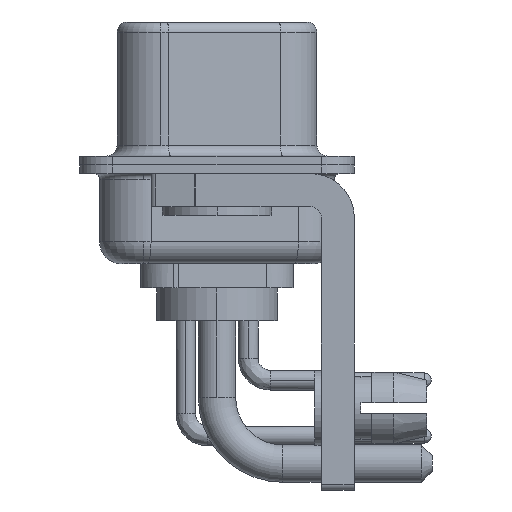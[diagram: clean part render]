
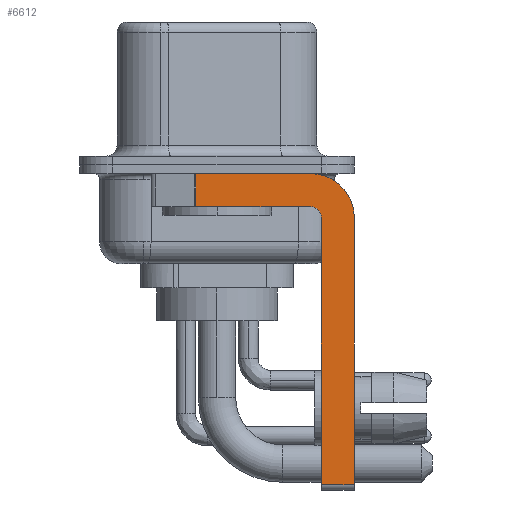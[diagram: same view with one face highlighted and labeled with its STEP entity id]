
A CAD part, left-side view. The second image highlights one B-rep face of the part: STEP entity #6612.
In plain terms, the highlighted planar face has unit normal (-1, 0, 0).
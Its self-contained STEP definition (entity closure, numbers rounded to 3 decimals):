
#338 = ORIENTED_EDGE ( 'NONE', *, *, #28988, .T. ) ;
#868 = VECTOR ( 'NONE', #25807, 1000. ) ;
#1048 = DIRECTION ( 'NONE',  ( 0., -1., 0. ) ) ;
#1994 = DIRECTION ( 'NONE',  ( 0., 0., -1. ) ) ;
#2663 = VERTEX_POINT ( 'NONE', #24443 ) ;
#2701 = CIRCLE ( 'NONE', #30660, 0.5 ) ;
#2788 = LINE ( 'NONE', #29220, #6670 ) ;
#3777 = CARTESIAN_POINT ( 'NONE',  ( -2.9, -4.25, -2.4 ) ) ;
#4065 = CARTESIAN_POINT ( 'NONE',  ( -2.9, -4.25, -1.9 ) ) ;
#4340 = ORIENTED_EDGE ( 'NONE', *, *, #30450, .F. ) ;
#4348 = VECTOR ( 'NONE', #19993, 1000. ) ;
#4601 = CARTESIAN_POINT ( 'NONE',  ( -2.9, -4.25, -0.4 ) ) ;
#5052 = CARTESIAN_POINT ( 'NONE',  ( -2.9, -4.25, -2.4 ) ) ;
#5652 = CIRCLE ( 'NONE', #23116, 2. ) ;
#6239 = DIRECTION ( 'NONE',  ( 1., 0., 0. ) ) ;
#6262 = VERTEX_POINT ( 'NONE', #14786 ) ;
#6302 = VERTEX_POINT ( 'NONE', #29773 ) ;
#6612 = ADVANCED_FACE ( 'NONE', ( #21775 ), #26008, .F. ) ;
#6670 = VECTOR ( 'NONE', #12960, 1000. ) ;
#8098 = LINE ( 'NONE', #15150, #29184 ) ;
#8377 = CARTESIAN_POINT ( 'NONE',  ( -2.9, -6.25, -2.4 ) ) ;
#8715 = ORIENTED_EDGE ( 'NONE', *, *, #28259, .F. ) ;
#8786 = DIRECTION ( 'NONE',  ( -1., 0., 0. ) ) ;
#9657 = VERTEX_POINT ( 'NONE', #15737 ) ;
#11607 = VECTOR ( 'NONE', #11825, 1000. ) ;
#11825 = DIRECTION ( 'NONE',  ( 0., 0., -1. ) ) ;
#11915 = DIRECTION ( 'NONE',  ( 0., 0., 1. ) ) ;
#12555 = CARTESIAN_POINT ( 'NONE',  ( -2.9, 0.978, -1.9 ) ) ;
#12960 = DIRECTION ( 'NONE',  ( 0., 0., -1. ) ) ;
#13123 = CARTESIAN_POINT ( 'NONE',  ( -2.9, -4.75, -14.8 ) ) ;
#13683 = ORIENTED_EDGE ( 'NONE', *, *, #20551, .T. ) ;
#14695 = DIRECTION ( 'NONE',  ( 0., -1., 0. ) ) ;
#14786 = CARTESIAN_POINT ( 'NONE',  ( -2.9, 0.978, -1.9 ) ) ;
#15150 = CARTESIAN_POINT ( 'NONE',  ( -2.9, 3., -0.4 ) ) ;
#15737 = CARTESIAN_POINT ( 'NONE',  ( -2.9, -4.25, -1.9 ) ) ;
#15927 = VERTEX_POINT ( 'NONE', #8377 ) ;
#16011 = EDGE_CURVE ( 'NONE', #9657, #6262, #25489, .T. ) ;
#16141 = CARTESIAN_POINT ( 'NONE',  ( -2.9, -6.25, -14.55 ) ) ;
#16448 = EDGE_CURVE ( 'NONE', #6302, #2663, #24690, .T. ) ;
#17642 = CARTESIAN_POINT ( 'NONE',  ( -2.9, -4.25, -14.55 ) ) ;
#18963 = DIRECTION ( 'NONE',  ( 1., 0., 0. ) ) ;
#19993 = DIRECTION ( 'NONE',  ( 0., 0., 1. ) ) ;
#20482 = VECTOR ( 'NONE', #1048, 1000. ) ;
#20551 = EDGE_CURVE ( 'NONE', #6302, #25291, #25135, .T. ) ;
#21337 = VERTEX_POINT ( 'NONE', #4601 ) ;
#21468 = DIRECTION ( 'NONE',  ( 0., 0., -1. ) ) ;
#21503 = ORIENTED_EDGE ( 'NONE', *, *, #25377, .F. ) ;
#21775 = FACE_OUTER_BOUND ( 'NONE', #22933, .T. ) ;
#22260 = CARTESIAN_POINT ( 'NONE',  ( -2.9, 0.978, -0.4 ) ) ;
#22804 = CARTESIAN_POINT ( 'NONE',  ( -2.9, -4.25, -2.4 ) ) ;
#22933 = EDGE_LOOP ( 'NONE', ( #29993, #338, #24516, #21503, #29927, #13683, #4340, #8715 ) ) ;
#23116 = AXIS2_PLACEMENT_3D ( 'NONE', #22804, #6239, #1994 ) ;
#24443 = CARTESIAN_POINT ( 'NONE',  ( -2.9, -4.75, -2.4 ) ) ;
#24516 = ORIENTED_EDGE ( 'NONE', *, *, #16011, .F. ) ;
#24690 = LINE ( 'NONE', #13123, #4348 ) ;
#25135 = LINE ( 'NONE', #17642, #20482 ) ;
#25291 = VERTEX_POINT ( 'NONE', #16141 ) ;
#25377 = EDGE_CURVE ( 'NONE', #2663, #9657, #2701, .T. ) ;
#25408 = AXIS2_PLACEMENT_3D ( 'NONE', #5052, #18963, #21468 ) ;
#25489 = LINE ( 'NONE', #4065, #868 ) ;
#25807 = DIRECTION ( 'NONE',  ( 0., 1., 0. ) ) ;
#26008 = PLANE ( 'NONE',  #25408 ) ;
#27222 = VERTEX_POINT ( 'NONE', #22260 ) ;
#28259 = EDGE_CURVE ( 'NONE', #21337, #15927, #5652, .T. ) ;
#28988 = EDGE_CURVE ( 'NONE', #27222, #6262, #30595, .T. ) ;
#29184 = VECTOR ( 'NONE', #14695, 1000. ) ;
#29220 = CARTESIAN_POINT ( 'NONE',  ( -2.9, -6.25, -2.4 ) ) ;
#29773 = CARTESIAN_POINT ( 'NONE',  ( -2.9, -4.75, -14.55 ) ) ;
#29927 = ORIENTED_EDGE ( 'NONE', *, *, #16448, .F. ) ;
#29993 = ORIENTED_EDGE ( 'NONE', *, *, #30552, .F. ) ;
#30450 = EDGE_CURVE ( 'NONE', #15927, #25291, #2788, .T. ) ;
#30552 = EDGE_CURVE ( 'NONE', #27222, #21337, #8098, .T. ) ;
#30595 = LINE ( 'NONE', #12555, #11607 ) ;
#30660 = AXIS2_PLACEMENT_3D ( 'NONE', #3777, #8786, #11915 ) ;
